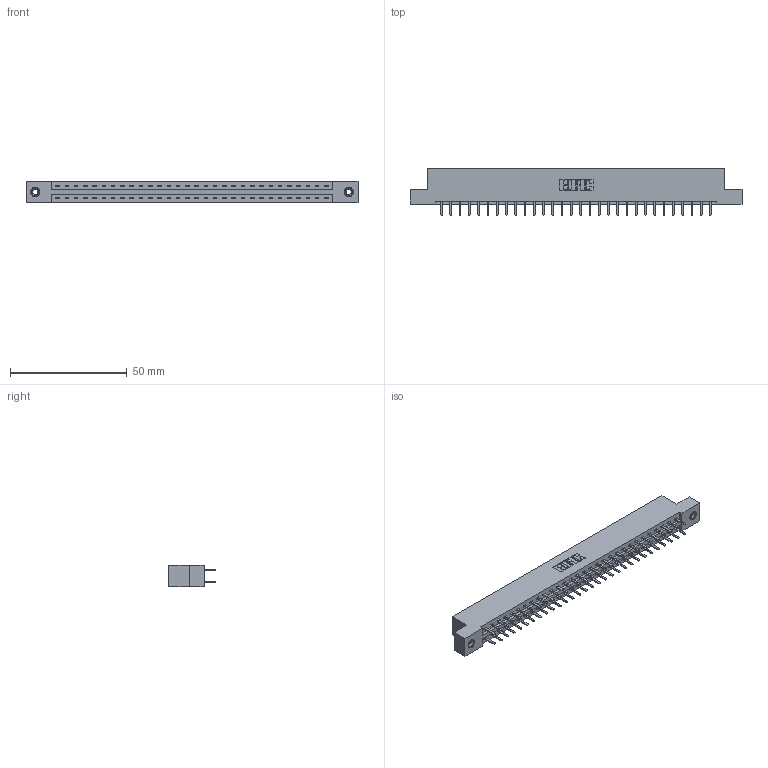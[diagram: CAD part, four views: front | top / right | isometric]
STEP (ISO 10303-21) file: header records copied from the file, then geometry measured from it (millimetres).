
FILE_DESCRIPTION (( 'STEP AP203' ), '1' );
FILE_NAME ('387-060-520-208.STEP', '2018-09-21T02:38:12', ( '' ), ( '' ), 'SwSTEP 2.0', 'SolidWorks 2016', '' );
FILE_SCHEMA (( 'CONFIG_CONTROL_DESIGN' ));
Length unit declared in the file: inch
Products named in the file (4): 337 Part_Flush Mounting Lugs - 0.156 Dia-TI; 345-292-001_345-293-120; 345-250-001_345-250-003-102; 387-060-520-208
Assembly tree (63 placements, depth 2):
  387-060-520-208
    337 Part_Flush Mounting Lugs - 0.156 Dia-TI
    345-292-001_345-293-120  x60
    345-250-001_345-250-003-102  x2
Bounding box: 141.88 x 20.02 x 9.4 mm (x, y, z)
Volume: 14760.3 mm3; surface area: 16518.7 mm2
Topology: 63 solids, 63 shells, 3654 faces, 10587 edges, 6890 vertices
Faces by surface type: plane 2502, cylinder 1136, cone 12, torus 4
Entity records: 26112 total; most frequent: CARTESIAN_POINT 4401, ORIENTED_EDGE 4318, DIRECTION 3785, EDGE_CURVE 2159, VECTOR 2007, LINE 2007, VERTEX_POINT 1432, AXIS2_PLACEMENT_3D 889
